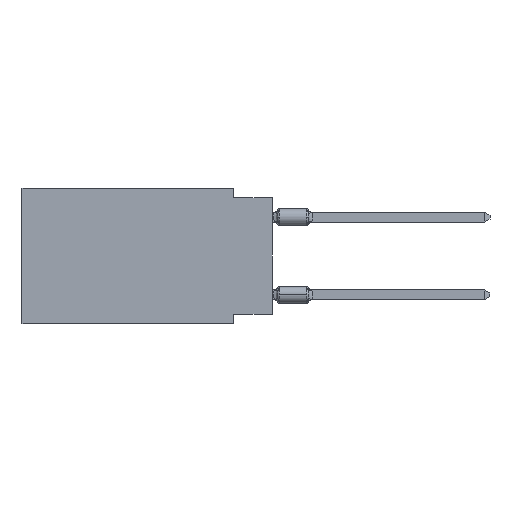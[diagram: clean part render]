
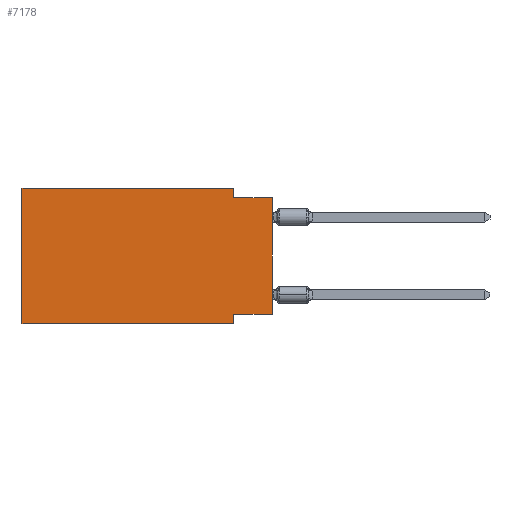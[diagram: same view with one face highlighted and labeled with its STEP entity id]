
A CAD part, left-side view. The second image highlights one B-rep face of the part: STEP entity #7178.
In plain terms, the highlighted planar face has unit normal (-1, 0, 0).
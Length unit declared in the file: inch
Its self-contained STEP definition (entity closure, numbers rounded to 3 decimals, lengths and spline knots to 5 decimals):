
#549 = LINE ( 'NONE', #14712, #634 ) ;
#634 = VECTOR ( 'NONE', #10976, 39.37008 ) ;
#1079 = EDGE_CURVE ( 'NONE', #1808, #10440, #1445, .T. ) ;
#1358 = EDGE_CURVE ( 'NONE', #10440, #4523, #14278, .T. ) ;
#1445 = LINE ( 'NONE', #6135, #3452 ) ;
#1641 = VECTOR ( 'NONE', #11502, 39.37008 ) ;
#1808 = VERTEX_POINT ( 'NONE', #7182 ) ;
#1899 = VECTOR ( 'NONE', #6875, 39.37008 ) ;
#2758 = VERTEX_POINT ( 'NONE', #8960 ) ;
#3039 = CARTESIAN_POINT ( 'NONE',  ( 0., 0.1, -0.35 ) ) ;
#3043 = ORIENTED_EDGE ( 'NONE', *, *, #14947, .T. ) ;
#3452 = VECTOR ( 'NONE', #10804, 39.37008 ) ;
#4265 = ORIENTED_EDGE ( 'NONE', *, *, #8047, .F. ) ;
#4523 = VERTEX_POINT ( 'NONE', #12184 ) ;
#4692 = CARTESIAN_POINT ( 'NONE',  ( 0., 0.645, -0.35 ) ) ;
#4720 = CARTESIAN_POINT ( 'NONE',  ( 0., 0.645, -0.35 ) ) ;
#4739 = ORIENTED_EDGE ( 'NONE', *, *, #1079, .F. ) ;
#4933 = AXIS2_PLACEMENT_3D ( 'NONE', #10644, #8211, #9124 ) ;
#4961 = ORIENTED_EDGE ( 'NONE', *, *, #11618, .F. ) ;
#5186 = ORIENTED_EDGE ( 'NONE', *, *, #1358, .F. ) ;
#5263 = LINE ( 'NONE', #13431, #6785 ) ;
#5344 = ORIENTED_EDGE ( 'NONE', *, *, #13280, .F. ) ;
#5371 = CARTESIAN_POINT ( 'NONE',  ( 0., 0.1, -0.325 ) ) ;
#5569 = DIRECTION ( 'NONE',  ( 0., 0., -1. ) ) ;
#5585 = PLANE ( 'NONE',  #4933 ) ;
#5744 = CARTESIAN_POINT ( 'NONE',  ( 0., 0., 0. ) ) ;
#5858 = LINE ( 'NONE', #4692, #1899 ) ;
#6121 = VECTOR ( 'NONE', #12078, 39.37008 ) ;
#6135 = CARTESIAN_POINT ( 'NONE',  ( 0., 0.645, 0. ) ) ;
#6155 = LINE ( 'NONE', #8689, #6121 ) ;
#6390 = VECTOR ( 'NONE', #14195, 39.37008 ) ;
#6661 = LINE ( 'NONE', #3039, #11375 ) ;
#6682 = VERTEX_POINT ( 'NONE', #5371 ) ;
#6785 = VECTOR ( 'NONE', #13352, 39.37008 ) ;
#6875 = DIRECTION ( 'NONE',  ( 0., -1., 0. ) ) ;
#7178 = ADVANCED_FACE ( 'NONE', ( #12597 ), #5585, .F. ) ;
#7182 = CARTESIAN_POINT ( 'NONE',  ( 0., 0.645, 0. ) ) ;
#7817 = EDGE_CURVE ( 'NONE', #9533, #1808, #549, .T. ) ;
#7840 = LINE ( 'NONE', #5744, #1641 ) ;
#8047 = EDGE_CURVE ( 'NONE', #4523, #9506, #5263, .T. ) ;
#8088 = CARTESIAN_POINT ( 'NONE',  ( 0., 0.1, -0.35 ) ) ;
#8211 = DIRECTION ( 'NONE',  ( 1., 0., 0. ) ) ;
#8689 = CARTESIAN_POINT ( 'NONE',  ( 0., 0., -0.325 ) ) ;
#8960 = CARTESIAN_POINT ( 'NONE',  ( 0., 0., -0.325 ) ) ;
#9124 = DIRECTION ( 'NONE',  ( 0., 0., -1. ) ) ;
#9180 = ORIENTED_EDGE ( 'NONE', *, *, #14133, .T. ) ;
#9506 = VERTEX_POINT ( 'NONE', #14763 ) ;
#9533 = VERTEX_POINT ( 'NONE', #4720 ) ;
#10440 = VERTEX_POINT ( 'NONE', #14546 ) ;
#10644 = CARTESIAN_POINT ( 'NONE',  ( 0., 0.645, 0. ) ) ;
#10716 = CARTESIAN_POINT ( 'NONE',  ( 0., 0.1, 0. ) ) ;
#10804 = DIRECTION ( 'NONE',  ( 0., -1., 0. ) ) ;
#10976 = DIRECTION ( 'NONE',  ( 0., 0., 1. ) ) ;
#11375 = VECTOR ( 'NONE', #5569, 39.37008 ) ;
#11502 = DIRECTION ( 'NONE',  ( 0., 0., 1. ) ) ;
#11618 = EDGE_CURVE ( 'NONE', #2758, #6682, #6155, .T. ) ;
#12078 = DIRECTION ( 'NONE',  ( 0., 1., 0. ) ) ;
#12184 = CARTESIAN_POINT ( 'NONE',  ( 0., 0.1, -0.025 ) ) ;
#12420 = VERTEX_POINT ( 'NONE', #8088 ) ;
#12597 = FACE_OUTER_BOUND ( 'NONE', #13997, .T. ) ;
#13280 = EDGE_CURVE ( 'NONE', #6682, #12420, #6661, .T. ) ;
#13352 = DIRECTION ( 'NONE',  ( 0., -1., 0. ) ) ;
#13431 = CARTESIAN_POINT ( 'NONE',  ( 0., 0., -0.025 ) ) ;
#13949 = ORIENTED_EDGE ( 'NONE', *, *, #7817, .F. ) ;
#13997 = EDGE_LOOP ( 'NONE', ( #9180, #4265, #5186, #4739, #13949, #3043, #5344, #4961 ) ) ;
#14133 = EDGE_CURVE ( 'NONE', #2758, #9506, #7840, .T. ) ;
#14195 = DIRECTION ( 'NONE',  ( 0., 0., -1. ) ) ;
#14278 = LINE ( 'NONE', #10716, #6390 ) ;
#14546 = CARTESIAN_POINT ( 'NONE',  ( 0., 0.1, 0. ) ) ;
#14712 = CARTESIAN_POINT ( 'NONE',  ( 0., 0.645, 0. ) ) ;
#14763 = CARTESIAN_POINT ( 'NONE',  ( 0., 0., -0.025 ) ) ;
#14947 = EDGE_CURVE ( 'NONE', #9533, #12420, #5858, .T. ) ;
